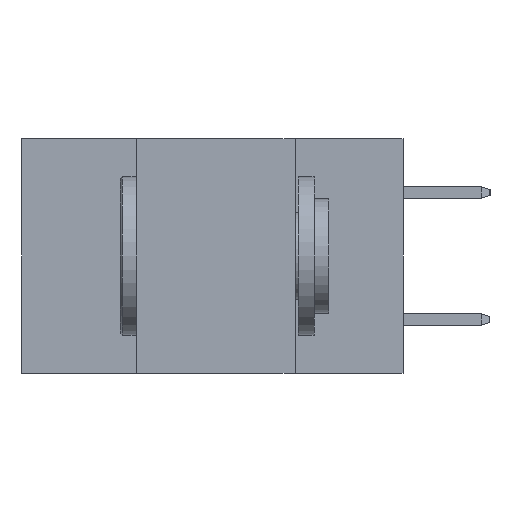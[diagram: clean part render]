
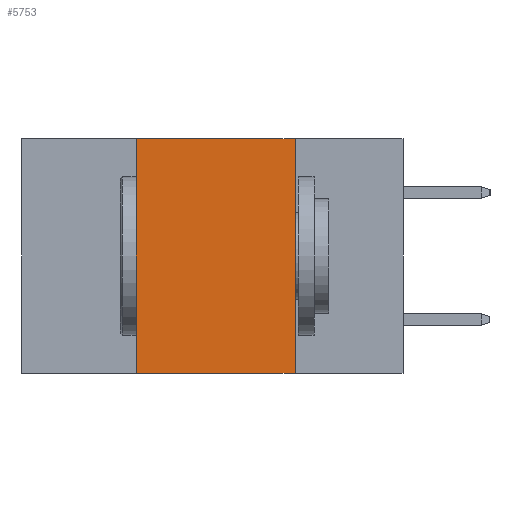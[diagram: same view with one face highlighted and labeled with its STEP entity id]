
A CAD part, left-side view. The second image highlights one B-rep face of the part: STEP entity #5753.
In plain terms, the highlighted planar face has unit normal (-1, 0, 0).
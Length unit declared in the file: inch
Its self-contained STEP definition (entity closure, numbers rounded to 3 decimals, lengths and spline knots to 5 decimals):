
#85 = VECTOR ( 'NONE', #2680, 39.37008 ) ;
#248 = CARTESIAN_POINT ( 'NONE',  ( 0., 0.17, -0.37 ) ) ;
#395 = PLANE ( 'NONE',  #6403 ) ;
#566 = VECTOR ( 'NONE', #5963, 39.37008 ) ;
#578 = EDGE_CURVE ( 'NONE', #3268, #7770, #2737, .T. ) ;
#934 = CARTESIAN_POINT ( 'NONE',  ( 0., 0.42, -0.37 ) ) ;
#1702 = VECTOR ( 'NONE', #10112, 39.37008 ) ;
#1892 = CARTESIAN_POINT ( 'NONE',  ( 0., 0.42, 0. ) ) ;
#2680 = DIRECTION ( 'NONE',  ( 0., -1., 0. ) ) ;
#2737 = LINE ( 'NONE', #2910, #85 ) ;
#2909 = ORIENTED_EDGE ( 'NONE', *, *, #578, .F. ) ;
#2910 = CARTESIAN_POINT ( 'NONE',  ( 0., 0.6, 0. ) ) ;
#3268 = VERTEX_POINT ( 'NONE', #9570 ) ;
#3718 = ORIENTED_EDGE ( 'NONE', *, *, #6809, .F. ) ;
#4219 = EDGE_LOOP ( 'NONE', ( #3718, #2909, #8316, #9336 ) ) ;
#4267 = EDGE_CURVE ( 'NONE', #6064, #3268, #9997, .T. ) ;
#4420 = CARTESIAN_POINT ( 'NONE',  ( 0., 0.17, 0. ) ) ;
#4781 = DIRECTION ( 'NONE',  ( 1., 0., 0. ) ) ;
#4967 = LINE ( 'NONE', #8501, #566 ) ;
#5428 = DIRECTION ( 'NONE',  ( 0., 0., -1. ) ) ;
#5753 = ADVANCED_FACE ( 'NONE', ( #5900 ), #395, .F. ) ;
#5900 = FACE_OUTER_BOUND ( 'NONE', #4219, .T. ) ;
#5963 = DIRECTION ( 'NONE',  ( 0., -1., 0. ) ) ;
#6064 = VERTEX_POINT ( 'NONE', #934 ) ;
#6300 = LINE ( 'NONE', #4420, #6448 ) ;
#6395 = CARTESIAN_POINT ( 'NONE',  ( 0., 0.17, 0. ) ) ;
#6403 = AXIS2_PLACEMENT_3D ( 'NONE', #8552, #4781, #6775 ) ;
#6448 = VECTOR ( 'NONE', #5428, 39.37008 ) ;
#6723 = EDGE_CURVE ( 'NONE', #6064, #10737, #4967, .T. ) ;
#6775 = DIRECTION ( 'NONE',  ( 0., 0., -1. ) ) ;
#6809 = EDGE_CURVE ( 'NONE', #7770, #10737, #6300, .T. ) ;
#7770 = VERTEX_POINT ( 'NONE', #6395 ) ;
#8316 = ORIENTED_EDGE ( 'NONE', *, *, #4267, .F. ) ;
#8501 = CARTESIAN_POINT ( 'NONE',  ( 0., 0.6, -0.37 ) ) ;
#8552 = CARTESIAN_POINT ( 'NONE',  ( 0., 0.6, 0. ) ) ;
#9336 = ORIENTED_EDGE ( 'NONE', *, *, #6723, .T. ) ;
#9570 = CARTESIAN_POINT ( 'NONE',  ( 0., 0.42, 0. ) ) ;
#9997 = LINE ( 'NONE', #1892, #1702 ) ;
#10112 = DIRECTION ( 'NONE',  ( 0., 0., 1. ) ) ;
#10737 = VERTEX_POINT ( 'NONE', #248 ) ;
